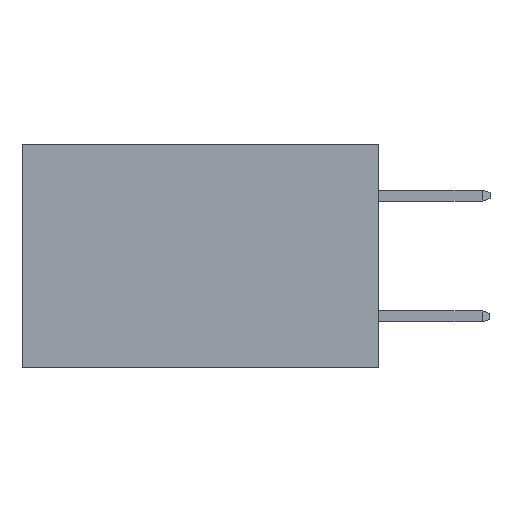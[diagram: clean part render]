
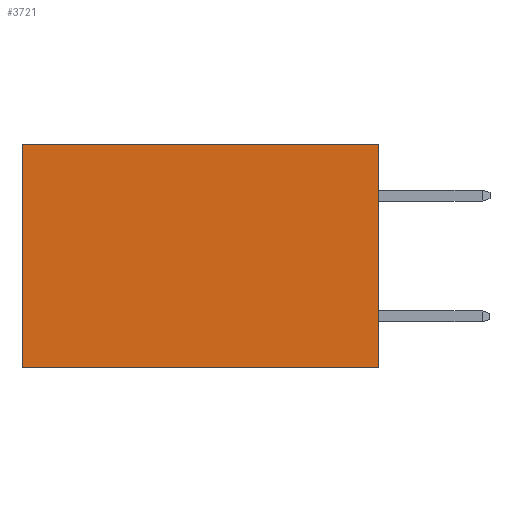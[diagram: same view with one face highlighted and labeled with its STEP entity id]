
A CAD part, left-side view. The second image highlights one B-rep face of the part: STEP entity #3721.
In plain terms, the highlighted planar face has unit normal (-1, 0, 0).
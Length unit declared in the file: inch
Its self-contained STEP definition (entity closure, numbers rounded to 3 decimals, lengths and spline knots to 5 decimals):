
#740 = VERTEX_POINT ( 'NONE', #6735 ) ;
#787 = VERTEX_POINT ( 'NONE', #5205 ) ;
#985 = EDGE_CURVE ( 'NONE', #1229, #6593, #6834, .T. ) ;
#1164 = EDGE_CURVE ( 'NONE', #740, #787, #4659, .T. ) ;
#1229 = VERTEX_POINT ( 'NONE', #1285 ) ;
#1285 = CARTESIAN_POINT ( 'NONE',  ( 0.277, 0.59, 0. ) ) ;
#1509 = DIRECTION ( 'NONE',  ( 0., 0., -1. ) ) ;
#1578 = CARTESIAN_POINT ( 'NONE',  ( 0.277, 0., -0.37 ) ) ;
#1887 = EDGE_CURVE ( 'NONE', #787, #6593, #3836, .T. ) ;
#1984 = ORIENTED_EDGE ( 'NONE', *, *, #985, .T. ) ;
#3161 = CARTESIAN_POINT ( 'NONE',  ( 0.277, 0., -0.37 ) ) ;
#3261 = DIRECTION ( 'NONE',  ( 0., 1., 0. ) ) ;
#3318 = CARTESIAN_POINT ( 'NONE',  ( 0.277, 0., 0. ) ) ;
#3430 = AXIS2_PLACEMENT_3D ( 'NONE', #6894, #6763, #6756 ) ;
#3721 = ADVANCED_FACE ( 'NONE', ( #7039 ), #6778, .F. ) ;
#3836 = LINE ( 'NONE', #3161, #5174 ) ;
#3961 = VECTOR ( 'NONE', #4206, 39.37008 ) ;
#4073 = CARTESIAN_POINT ( 'NONE',  ( 0.277, 0.59, -0.37 ) ) ;
#4206 = DIRECTION ( 'NONE',  ( 0., 0., -1. ) ) ;
#4659 = LINE ( 'NONE', #1578, #7525 ) ;
#4715 = ORIENTED_EDGE ( 'NONE', *, *, #6865, .T. ) ;
#5060 = ORIENTED_EDGE ( 'NONE', *, *, #1164, .F. ) ;
#5118 = DIRECTION ( 'NONE',  ( 0., 1., 0. ) ) ;
#5174 = VECTOR ( 'NONE', #5118, 39.37008 ) ;
#5205 = CARTESIAN_POINT ( 'NONE',  ( 0.277, 0., -0.37 ) ) ;
#5412 = ORIENTED_EDGE ( 'NONE', *, *, #1887, .F. ) ;
#5543 = LINE ( 'NONE', #3318, #5705 ) ;
#5705 = VECTOR ( 'NONE', #3261, 39.37008 ) ;
#6593 = VERTEX_POINT ( 'NONE', #7336 ) ;
#6735 = CARTESIAN_POINT ( 'NONE',  ( 0.277, 0., 0. ) ) ;
#6756 = DIRECTION ( 'NONE',  ( 0., 0., -1. ) ) ;
#6763 = DIRECTION ( 'NONE',  ( 1., 0., 0. ) ) ;
#6778 = PLANE ( 'NONE',  #3430 ) ;
#6794 = EDGE_LOOP ( 'NONE', ( #1984, #5412, #5060, #4715 ) ) ;
#6834 = LINE ( 'NONE', #4073, #3961 ) ;
#6865 = EDGE_CURVE ( 'NONE', #740, #1229, #5543, .T. ) ;
#6894 = CARTESIAN_POINT ( 'NONE',  ( 0.277, 0., -0.37 ) ) ;
#7039 = FACE_OUTER_BOUND ( 'NONE', #6794, .T. ) ;
#7336 = CARTESIAN_POINT ( 'NONE',  ( 0.277, 0.59, -0.37 ) ) ;
#7525 = VECTOR ( 'NONE', #1509, 39.37008 ) ;
